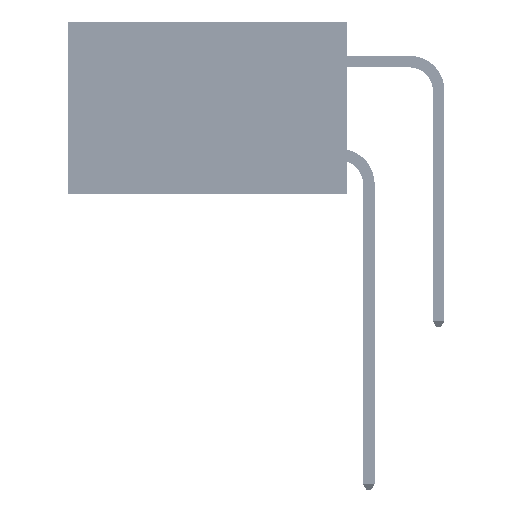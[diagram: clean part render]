
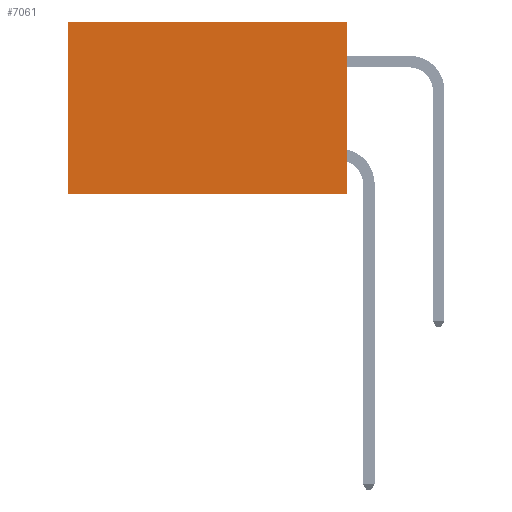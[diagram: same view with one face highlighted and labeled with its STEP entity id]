
A CAD part, left-side view. The second image highlights one B-rep face of the part: STEP entity #7061.
In plain terms, the highlighted planar face has unit normal (-1, 0, 0).
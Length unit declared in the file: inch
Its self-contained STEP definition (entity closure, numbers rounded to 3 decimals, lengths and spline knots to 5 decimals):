
#2015 = CARTESIAN_POINT ( 'NONE',  ( 0.2875, 0.6, 0. ) ) ;
#5818 = DIRECTION ( 'NONE',  ( 0., 0., -1. ) ) ;
#7061 = ADVANCED_FACE ( 'NONE', ( #36903 ), #46938, .F. ) ;
#8721 = CARTESIAN_POINT ( 'NONE',  ( 0.2875, 0.6, 0. ) ) ;
#8916 = LINE ( 'NONE', #8721, #48754 ) ;
#10305 = DIRECTION ( 'NONE',  ( 0., 1., 0. ) ) ;
#10473 = CARTESIAN_POINT ( 'NONE',  ( 0.2875, 0., 0. ) ) ;
#11503 = VECTOR ( 'NONE', #10305, 39.37008 ) ;
#13886 = ORIENTED_EDGE ( 'NONE', *, *, #25513, .F. ) ;
#16644 = VECTOR ( 'NONE', #21745, 39.37008 ) ;
#16916 = ORIENTED_EDGE ( 'NONE', *, *, #34626, .T. ) ;
#16950 = CARTESIAN_POINT ( 'NONE',  ( 0.2875, 0., 0. ) ) ;
#18562 = CARTESIAN_POINT ( 'NONE',  ( 0.2875, 0., -0.37 ) ) ;
#21058 = ORIENTED_EDGE ( 'NONE', *, *, #38447, .T. ) ;
#21745 = DIRECTION ( 'NONE',  ( 0., 1., 0. ) ) ;
#22406 = LINE ( 'NONE', #18562, #11503 ) ;
#22521 = VECTOR ( 'NONE', #49493, 39.37008 ) ;
#25050 = CARTESIAN_POINT ( 'NONE',  ( 0.2875, 0., 0. ) ) ;
#25513 = EDGE_CURVE ( 'NONE', #48386, #46549, #45660, .T. ) ;
#28989 = ORIENTED_EDGE ( 'NONE', *, *, #34850, .F. ) ;
#29129 = CARTESIAN_POINT ( 'NONE',  ( 0.2875, 0.6, -0.37 ) ) ;
#32419 = EDGE_LOOP ( 'NONE', ( #16916, #28989, #13886, #21058 ) ) ;
#32892 = AXIS2_PLACEMENT_3D ( 'NONE', #10473, #50899, #5818 ) ;
#34626 = EDGE_CURVE ( 'NONE', #40956, #44829, #8916, .T. ) ;
#34850 = EDGE_CURVE ( 'NONE', #46549, #44829, #22406, .T. ) ;
#36903 = FACE_OUTER_BOUND ( 'NONE', #32419, .T. ) ;
#37811 = LINE ( 'NONE', #46346, #16644 ) ;
#38447 = EDGE_CURVE ( 'NONE', #48386, #40956, #37811, .T. ) ;
#40956 = VERTEX_POINT ( 'NONE', #2015 ) ;
#41988 = CARTESIAN_POINT ( 'NONE',  ( 0.2875, 0., -0.37 ) ) ;
#44829 = VERTEX_POINT ( 'NONE', #29129 ) ;
#45660 = LINE ( 'NONE', #16950, #22521 ) ;
#45712 = DIRECTION ( 'NONE',  ( 0., 0., -1. ) ) ;
#46346 = CARTESIAN_POINT ( 'NONE',  ( 0.2875, 0., 0. ) ) ;
#46549 = VERTEX_POINT ( 'NONE', #41988 ) ;
#46938 = PLANE ( 'NONE',  #32892 ) ;
#48386 = VERTEX_POINT ( 'NONE', #25050 ) ;
#48754 = VECTOR ( 'NONE', #45712, 39.37008 ) ;
#49493 = DIRECTION ( 'NONE',  ( 0., 0., -1. ) ) ;
#50899 = DIRECTION ( 'NONE',  ( 1., 0., 0. ) ) ;
